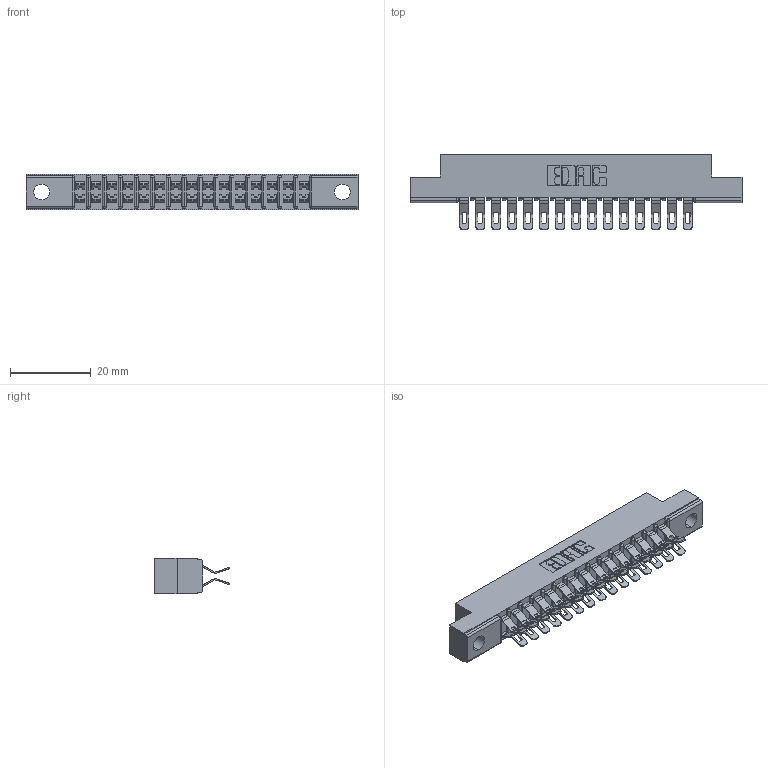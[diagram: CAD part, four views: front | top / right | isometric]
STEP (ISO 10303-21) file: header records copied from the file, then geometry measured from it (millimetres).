
FILE_DESCRIPTION (( 'STEP AP203' ), '1' );
FILE_NAME ('307-030-455-204.STEP', '2020-09-29T09:44:58', ( '' ), ( '' ), 'SwSTEP 2.0', 'SolidWorks 2020', '' );
FILE_SCHEMA (( 'CONFIG_CONTROL_DESIGN' ));
Length unit declared in the file: inch
Products named in the file (3): 307-030-455-204; 307-290-001_555; 307 Part_.156 Dia Mounting Holes
Assembly tree (31 placements, depth 2):
  307-030-455-204
    307 Part_.156 Dia Mounting Holes
    307-290-001_555  x30
Bounding box: 82.45 x 18.75 x 8.71 mm (x, y, z)
Volume: 5377.2 mm3; surface area: 9514.6 mm2
Topology: 31 solids, 31 shells, 1978 faces, 5789 edges, 3774 vertices
Faces by surface type: plane 1104, cylinder 842, sphere 32
Entity records: 17623 total; most frequent: CARTESIAN_POINT 2901, ORIENTED_EDGE 2872, DIRECTION 2852, EDGE_CURVE 1436, VECTOR 1086, LINE 1086, VERTEX_POINT 932, AXIS2_PLACEMENT_3D 883
